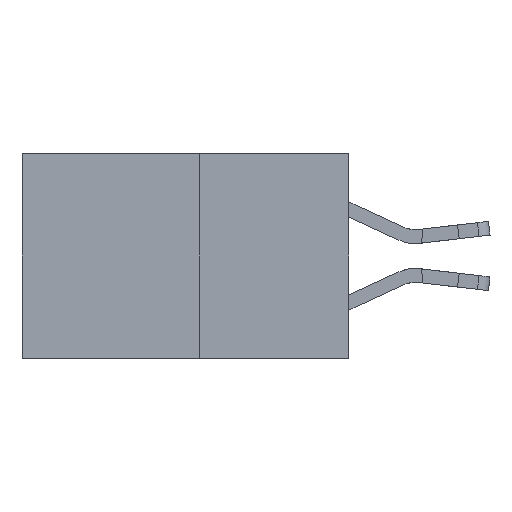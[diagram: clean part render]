
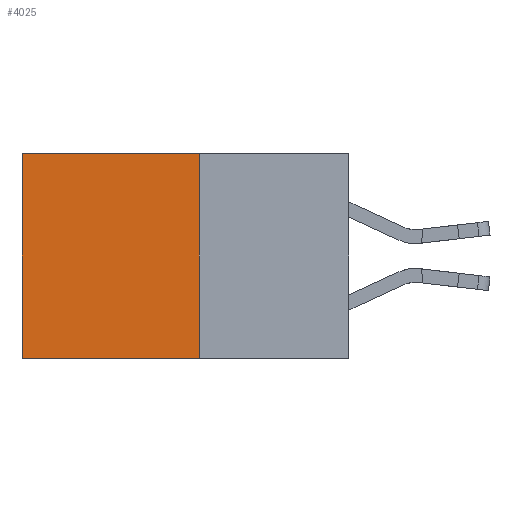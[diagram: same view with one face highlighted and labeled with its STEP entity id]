
A CAD part, left-side view. The second image highlights one B-rep face of the part: STEP entity #4025.
In plain terms, the highlighted planar face has unit normal (-1, 0, 0).
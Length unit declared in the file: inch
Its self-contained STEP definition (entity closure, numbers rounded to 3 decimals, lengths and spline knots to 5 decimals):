
#2635 = DIRECTION ( 'NONE',  ( 0., 1., 0. ) ) ;
#2651 = DIRECTION ( 'NONE',  ( 0., 0., -1. ) ) ;
#2882 = LINE ( 'NONE', #4687, #6070 ) ;
#3401 = AXIS2_PLACEMENT_3D ( 'NONE', #8185, #7764, #7057 ) ;
#3890 = VERTEX_POINT ( 'NONE', #9326 ) ;
#4025 = ADVANCED_FACE ( 'NONE', ( #12050 ), #8205, .F. ) ;
#4687 = CARTESIAN_POINT ( 'NONE',  ( 0.277, 0.27, -0.37 ) ) ;
#4991 = CARTESIAN_POINT ( 'NONE',  ( 0.277, 0.27, -0.37 ) ) ;
#5736 = VECTOR ( 'NONE', #2651, 39.37008 ) ;
#6070 = VECTOR ( 'NONE', #13902, 39.37008 ) ;
#6223 = VERTEX_POINT ( 'NONE', #4991 ) ;
#6299 = EDGE_CURVE ( 'NONE', #3890, #6223, #9704, .T. ) ;
#6934 = ORIENTED_EDGE ( 'NONE', *, *, #12053, .F. ) ;
#7057 = DIRECTION ( 'NONE',  ( 0., 0., -1. ) ) ;
#7158 = EDGE_LOOP ( 'NONE', ( #11104, #6934, #11723, #8959 ) ) ;
#7764 = DIRECTION ( 'NONE',  ( 1., 0., 0. ) ) ;
#8185 = CARTESIAN_POINT ( 'NONE',  ( 0.277, 0.27, -0.37 ) ) ;
#8205 = PLANE ( 'NONE',  #3401 ) ;
#8484 = LINE ( 'NONE', #9270, #15386 ) ;
#8959 = ORIENTED_EDGE ( 'NONE', *, *, #14365, .T. ) ;
#8984 = VERTEX_POINT ( 'NONE', #10063 ) ;
#9258 = EDGE_CURVE ( 'NONE', #16132, #8984, #12789, .T. ) ;
#9270 = CARTESIAN_POINT ( 'NONE',  ( 0.277, 0.27, 0. ) ) ;
#9326 = CARTESIAN_POINT ( 'NONE',  ( 0.277, 0.27, 0. ) ) ;
#9704 = LINE ( 'NONE', #16574, #16165 ) ;
#10063 = CARTESIAN_POINT ( 'NONE',  ( 0.277, 0.59, -0.37 ) ) ;
#10528 = CARTESIAN_POINT ( 'NONE',  ( 0.277, 0.59, 0. ) ) ;
#11104 = ORIENTED_EDGE ( 'NONE', *, *, #9258, .T. ) ;
#11723 = ORIENTED_EDGE ( 'NONE', *, *, #6299, .F. ) ;
#12003 = CARTESIAN_POINT ( 'NONE',  ( 0.277, 0.59, -0.37 ) ) ;
#12050 = FACE_OUTER_BOUND ( 'NONE', #7158, .T. ) ;
#12053 = EDGE_CURVE ( 'NONE', #6223, #8984, #2882, .T. ) ;
#12789 = LINE ( 'NONE', #12003, #5736 ) ;
#13902 = DIRECTION ( 'NONE',  ( 0., 1., 0. ) ) ;
#14365 = EDGE_CURVE ( 'NONE', #3890, #16132, #8484, .T. ) ;
#15386 = VECTOR ( 'NONE', #2635, 39.37008 ) ;
#15700 = DIRECTION ( 'NONE',  ( 0., 0., -1. ) ) ;
#16132 = VERTEX_POINT ( 'NONE', #10528 ) ;
#16165 = VECTOR ( 'NONE', #15700, 39.37008 ) ;
#16574 = CARTESIAN_POINT ( 'NONE',  ( 0.277, 0.27, -0.37 ) ) ;
